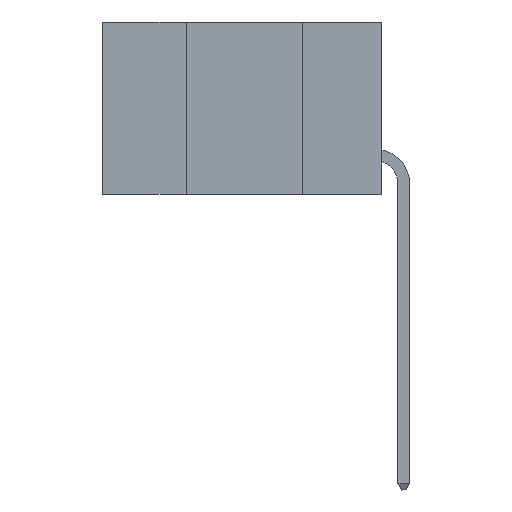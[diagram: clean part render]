
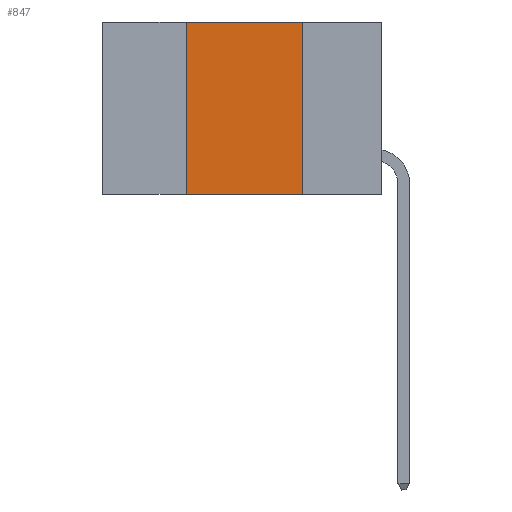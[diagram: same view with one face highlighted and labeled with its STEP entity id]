
A CAD part, left-side view. The second image highlights one B-rep face of the part: STEP entity #847.
In plain terms, the highlighted planar face has unit normal (-1, 0, 0).
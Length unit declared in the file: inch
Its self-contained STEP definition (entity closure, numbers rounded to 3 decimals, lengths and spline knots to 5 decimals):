
#401 = CARTESIAN_POINT ( 'NONE',  ( 0., 0.17, -0.37 ) ) ;
#688 = VECTOR ( 'NONE', #2060, 39.37008 ) ;
#758 = CARTESIAN_POINT ( 'NONE',  ( 0., 0.17, 0. ) ) ;
#847 = ADVANCED_FACE ( 'NONE', ( #9585 ), #4648, .F. ) ;
#919 = LINE ( 'NONE', #8291, #688 ) ;
#965 = VECTOR ( 'NONE', #4164, 39.37008 ) ;
#1225 = DIRECTION ( 'NONE',  ( 0., 0., -1. ) ) ;
#1375 = VERTEX_POINT ( 'NONE', #7705 ) ;
#1478 = ORIENTED_EDGE ( 'NONE', *, *, #3970, .F. ) ;
#1539 = DIRECTION ( 'NONE',  ( 0., 0., -1. ) ) ;
#1573 = CARTESIAN_POINT ( 'NONE',  ( 0., 0.42, 0. ) ) ;
#1632 = VECTOR ( 'NONE', #3775, 39.37008 ) ;
#2016 = LINE ( 'NONE', #1573, #1632 ) ;
#2060 = DIRECTION ( 'NONE',  ( 0., -1., 0. ) ) ;
#2583 = CARTESIAN_POINT ( 'NONE',  ( 0., 0.6, -0.37 ) ) ;
#3504 = CARTESIAN_POINT ( 'NONE',  ( 0., 0.17, 0. ) ) ;
#3587 = AXIS2_PLACEMENT_3D ( 'NONE', #4613, #6331, #1539 ) ;
#3699 = VECTOR ( 'NONE', #1225, 39.37008 ) ;
#3775 = DIRECTION ( 'NONE',  ( 0., 0., 1. ) ) ;
#3810 = VERTEX_POINT ( 'NONE', #758 ) ;
#3970 = EDGE_CURVE ( 'NONE', #1375, #7464, #2016, .T. ) ;
#4164 = DIRECTION ( 'NONE',  ( 0., -1., 0. ) ) ;
#4197 = VERTEX_POINT ( 'NONE', #401 ) ;
#4572 = ORIENTED_EDGE ( 'NONE', *, *, #6538, .T. ) ;
#4613 = CARTESIAN_POINT ( 'NONE',  ( 0., 0.6, 0. ) ) ;
#4648 = PLANE ( 'NONE',  #3587 ) ;
#4797 = EDGE_LOOP ( 'NONE', ( #7634, #6374, #1478, #4572 ) ) ;
#5048 = CARTESIAN_POINT ( 'NONE',  ( 0., 0.42, 0. ) ) ;
#6083 = EDGE_CURVE ( 'NONE', #3810, #4197, #10098, .T. ) ;
#6331 = DIRECTION ( 'NONE',  ( 1., 0., 0. ) ) ;
#6374 = ORIENTED_EDGE ( 'NONE', *, *, #8816, .F. ) ;
#6538 = EDGE_CURVE ( 'NONE', #1375, #4197, #8115, .T. ) ;
#7464 = VERTEX_POINT ( 'NONE', #5048 ) ;
#7634 = ORIENTED_EDGE ( 'NONE', *, *, #6083, .F. ) ;
#7705 = CARTESIAN_POINT ( 'NONE',  ( 0., 0.42, -0.37 ) ) ;
#8115 = LINE ( 'NONE', #2583, #965 ) ;
#8291 = CARTESIAN_POINT ( 'NONE',  ( 0., 0.6, 0. ) ) ;
#8816 = EDGE_CURVE ( 'NONE', #7464, #3810, #919, .T. ) ;
#9585 = FACE_OUTER_BOUND ( 'NONE', #4797, .T. ) ;
#10098 = LINE ( 'NONE', #3504, #3699 ) ;
